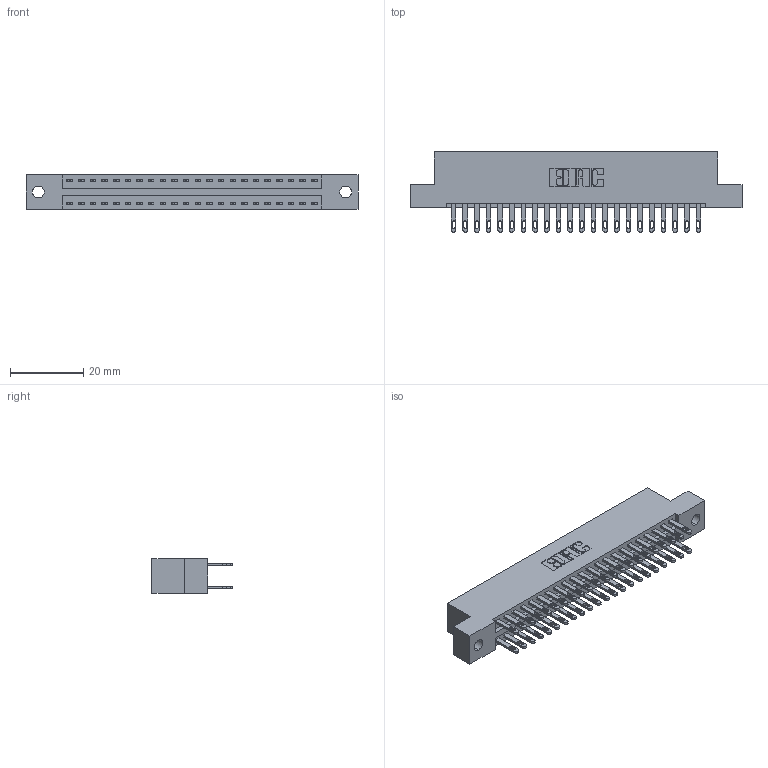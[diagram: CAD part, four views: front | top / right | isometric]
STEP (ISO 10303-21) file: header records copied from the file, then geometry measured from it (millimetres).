
FILE_DESCRIPTION (( 'STEP AP203' ), '1' );
FILE_NAME ('346-044-500-202.STEP', '2018-08-25T00:45:33', ( '' ), ( '' ), 'SwSTEP 2.0', 'SolidWorks 2016', '' );
FILE_SCHEMA (( 'CONFIG_CONTROL_DESIGN' ));
Length unit declared in the file: inch
Products named in the file (3): 345-292-001_345-293-100; 346-044-500-202; 346 Part_Flush Mounting Lugs - 0.128 Dia
Assembly tree (45 placements, depth 2):
  346-044-500-202
    346 Part_Flush Mounting Lugs - 0.128 Dia
    345-292-001_345-293-100  x44
Bounding box: 90.42 x 21.84 x 9.4 mm (x, y, z)
Volume: 8759.9 mm3; surface area: 11918 mm2
Topology: 45 solids, 45 shells, 2234 faces, 6797 edges, 4530 vertices
Faces by surface type: plane 1352, cylinder 882
Entity records: 16983 total; most frequent: CARTESIAN_POINT 2824, ORIENTED_EDGE 2758, DIRECTION 2543, EDGE_CURVE 1379, LINE 1155, VECTOR 1155, VERTEX_POINT 918, AXIS2_PLACEMENT_3D 694
